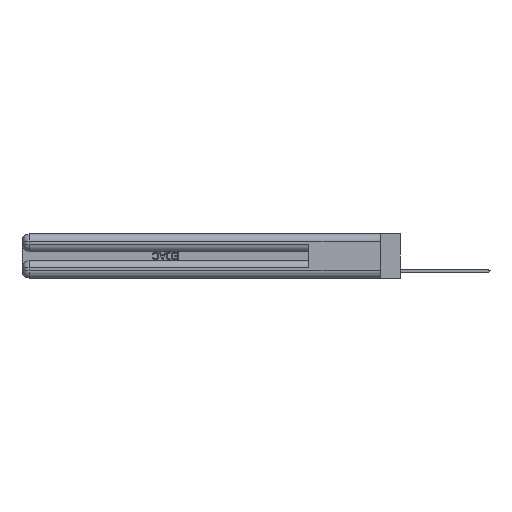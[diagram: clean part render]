
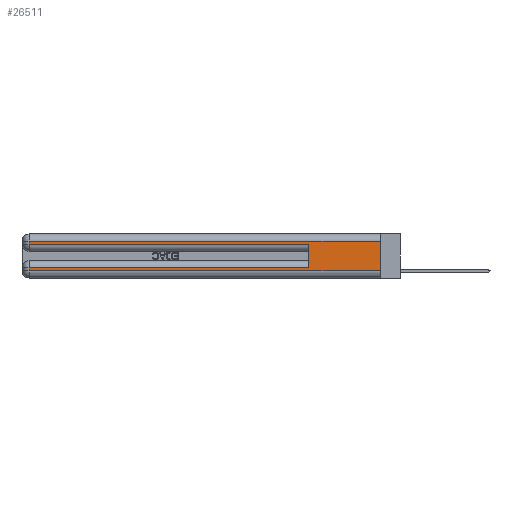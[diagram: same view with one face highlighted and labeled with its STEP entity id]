
A CAD part, left-side view. The second image highlights one B-rep face of the part: STEP entity #26511.
In plain terms, the highlighted planar face has unit normal (-1, 0, 0).
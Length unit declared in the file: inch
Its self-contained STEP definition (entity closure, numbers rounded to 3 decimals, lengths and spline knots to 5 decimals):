
#287 = VECTOR ( 'NONE', #12724, 39.37008 ) ;
#1294 = EDGE_CURVE ( 'NONE', #30465, #18818, #28918, .T. ) ;
#1320 = VERTEX_POINT ( 'NONE', #14555 ) ;
#3443 = DIRECTION ( 'NONE',  ( 1., 0., 0. ) ) ;
#3972 = LINE ( 'NONE', #6310, #5122 ) ;
#4110 = EDGE_LOOP ( 'NONE', ( #11199, #9480, #26895, #6935, #28871, #19153, #27120, #9406 ) ) ;
#4237 = DIRECTION ( 'NONE',  ( 0., 0., 1. ) ) ;
#4726 = VECTOR ( 'NONE', #15862, 39.37008 ) ;
#4877 = CARTESIAN_POINT ( 'NONE',  ( 0., 0., 0.31 ) ) ;
#5122 = VECTOR ( 'NONE', #13529, 39.37008 ) ;
#5687 = LINE ( 'NONE', #17084, #287 ) ;
#6165 = CARTESIAN_POINT ( 'NONE',  ( 0., 2.94, 0.37 ) ) ;
#6310 = CARTESIAN_POINT ( 'NONE',  ( 0., 0., 0.06 ) ) ;
#6481 = DIRECTION ( 'NONE',  ( 0., 0., -1. ) ) ;
#6935 = ORIENTED_EDGE ( 'NONE', *, *, #17222, .T. ) ;
#7251 = EDGE_CURVE ( 'NONE', #18533, #13965, #9148, .T. ) ;
#7995 = PLANE ( 'NONE',  #13614 ) ;
#8550 = LINE ( 'NONE', #15706, #4726 ) ;
#9148 = LINE ( 'NONE', #18654, #22184 ) ;
#9406 = ORIENTED_EDGE ( 'NONE', *, *, #26230, .T. ) ;
#9480 = ORIENTED_EDGE ( 'NONE', *, *, #1294, .T. ) ;
#10068 = DIRECTION ( 'NONE',  ( 0., -1., 0. ) ) ;
#10322 = VECTOR ( 'NONE', #4237, 39.37008 ) ;
#11033 = CARTESIAN_POINT ( 'NONE',  ( 0., 2.94, 0.06 ) ) ;
#11199 = ORIENTED_EDGE ( 'NONE', *, *, #28605, .F. ) ;
#11618 = EDGE_CURVE ( 'NONE', #13965, #28599, #28045, .T. ) ;
#11623 = CARTESIAN_POINT ( 'NONE',  ( 0., 2.94, 0.31 ) ) ;
#12108 = FACE_OUTER_BOUND ( 'NONE', #4110, .T. ) ;
#12119 = CARTESIAN_POINT ( 'NONE',  ( 0., 0., 0.285 ) ) ;
#12268 = CARTESIAN_POINT ( 'NONE',  ( 0., 0., 0.06 ) ) ;
#12724 = DIRECTION ( 'NONE',  ( 0., 0., -1. ) ) ;
#13529 = DIRECTION ( 'NONE',  ( 0., -1., 0. ) ) ;
#13614 = AXIS2_PLACEMENT_3D ( 'NONE', #27176, #3443, #17491 ) ;
#13625 = LINE ( 'NONE', #20628, #10322 ) ;
#13861 = VERTEX_POINT ( 'NONE', #12268 ) ;
#13965 = VERTEX_POINT ( 'NONE', #20663 ) ;
#13987 = DIRECTION ( 'NONE',  ( 0., 1., 0. ) ) ;
#14555 = CARTESIAN_POINT ( 'NONE',  ( 0., 0.6, 0.285 ) ) ;
#15706 = CARTESIAN_POINT ( 'NONE',  ( 0., 0., 0.37 ) ) ;
#15862 = DIRECTION ( 'NONE',  ( 0., 0., -1. ) ) ;
#16755 = DIRECTION ( 'NONE',  ( 0., 1., 0. ) ) ;
#17084 = CARTESIAN_POINT ( 'NONE',  ( 0., 2.94, 0.37 ) ) ;
#17222 = EDGE_CURVE ( 'NONE', #30116, #1320, #26452, .T. ) ;
#17491 = DIRECTION ( 'NONE',  ( 0., 0., -1. ) ) ;
#17715 = VECTOR ( 'NONE', #16755, 39.37008 ) ;
#18533 = VERTEX_POINT ( 'NONE', #28964 ) ;
#18654 = CARTESIAN_POINT ( 'NONE',  ( 0., 0., 0.085 ) ) ;
#18818 = VERTEX_POINT ( 'NONE', #11623 ) ;
#19153 = ORIENTED_EDGE ( 'NONE', *, *, #7251, .T. ) ;
#20628 = CARTESIAN_POINT ( 'NONE',  ( 0., 0.6, 0.145 ) ) ;
#20663 = CARTESIAN_POINT ( 'NONE',  ( 0., 2.94, 0.085 ) ) ;
#21416 = EDGE_CURVE ( 'NONE', #18533, #1320, #13625, .T. ) ;
#22184 = VECTOR ( 'NONE', #13987, 39.37008 ) ;
#25102 = CARTESIAN_POINT ( 'NONE',  ( 0., 2.94, 0.285 ) ) ;
#25409 = VECTOR ( 'NONE', #10068, 39.37008 ) ;
#26230 = EDGE_CURVE ( 'NONE', #28599, #13861, #3972, .T. ) ;
#26329 = VECTOR ( 'NONE', #6481, 39.37008 ) ;
#26452 = LINE ( 'NONE', #12119, #25409 ) ;
#26511 = ADVANCED_FACE ( 'NONE', ( #12108 ), #7995, .F. ) ;
#26895 = ORIENTED_EDGE ( 'NONE', *, *, #29481, .T. ) ;
#27120 = ORIENTED_EDGE ( 'NONE', *, *, #11618, .T. ) ;
#27176 = CARTESIAN_POINT ( 'NONE',  ( 0., 0., 0.37 ) ) ;
#28045 = LINE ( 'NONE', #6165, #26329 ) ;
#28599 = VERTEX_POINT ( 'NONE', #11033 ) ;
#28605 = EDGE_CURVE ( 'NONE', #30465, #13861, #8550, .T. ) ;
#28871 = ORIENTED_EDGE ( 'NONE', *, *, #21416, .F. ) ;
#28918 = LINE ( 'NONE', #4877, #17715 ) ;
#28964 = CARTESIAN_POINT ( 'NONE',  ( 0., 0.6, 0.085 ) ) ;
#29162 = CARTESIAN_POINT ( 'NONE',  ( 0., 0., 0.31 ) ) ;
#29481 = EDGE_CURVE ( 'NONE', #18818, #30116, #5687, .T. ) ;
#30116 = VERTEX_POINT ( 'NONE', #25102 ) ;
#30465 = VERTEX_POINT ( 'NONE', #29162 ) ;
